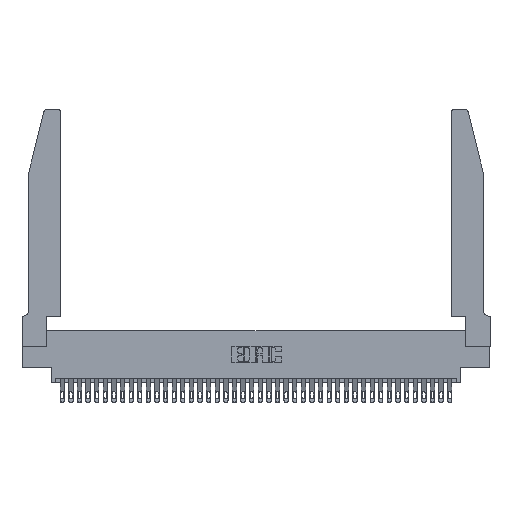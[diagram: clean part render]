
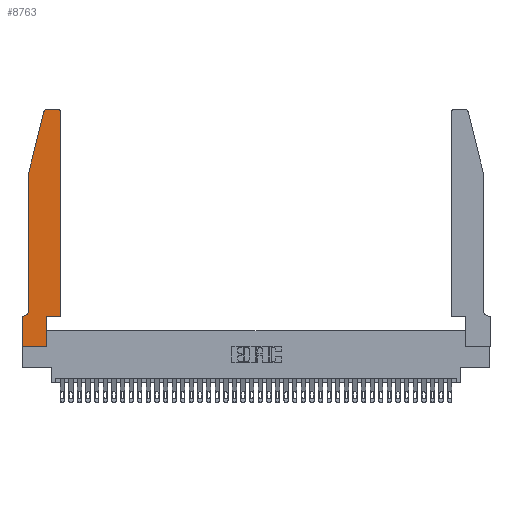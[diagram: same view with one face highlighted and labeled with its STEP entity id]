
A CAD part, top view. The second image highlights one B-rep face of the part: STEP entity #8763.
In plain terms, the highlighted planar face has unit normal (0, 0, 1).
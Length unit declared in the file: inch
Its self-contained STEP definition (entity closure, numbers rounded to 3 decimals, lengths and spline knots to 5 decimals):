
#928 = CARTESIAN_POINT ( 'NONE',  ( 0., 0., 0.37 ) ) ;
#1356 = DIRECTION ( 'NONE',  ( 0., 0., -1. ) ) ;
#1429 = CARTESIAN_POINT ( 'NONE',  ( 0.4505, 0.35, 0.37 ) ) ;
#1814 = EDGE_CURVE ( 'NONE', #34689, #28188, #25560, .T. ) ;
#1971 = AXIS2_PLACEMENT_3D ( 'NONE', #34508, #29140, #38449 ) ;
#2319 = CARTESIAN_POINT ( 'NONE',  ( 0.0755, 0.42, 0.37 ) ) ;
#2362 = VERTEX_POINT ( 'NONE', #7600 ) ;
#2422 = VECTOR ( 'NONE', #18230, 39.37008 ) ;
#2549 = DIRECTION ( 'NONE',  ( 1., 0., 0. ) ) ;
#3381 = ORIENTED_EDGE ( 'NONE', *, *, #33656, .T. ) ;
#3677 = CARTESIAN_POINT ( 'NONE',  ( 0.0755, 2., 0.37 ) ) ;
#3702 = LINE ( 'NONE', #26483, #21016 ) ;
#3932 = VERTEX_POINT ( 'NONE', #34765 ) ;
#4881 = DIRECTION ( 'NONE',  ( 0., -1., 0. ) ) ;
#5626 = LINE ( 'NONE', #1429, #12023 ) ;
#5709 = CARTESIAN_POINT ( 'NONE',  ( 0.4505, 0.35, 0.37 ) ) ;
#5847 = LINE ( 'NONE', #13348, #21200 ) ;
#5885 = CARTESIAN_POINT ( 'NONE',  ( 0., 0., 0.37 ) ) ;
#6052 = CARTESIAN_POINT ( 'NONE',  ( 0.4505, 2.72, 0.37 ) ) ;
#7284 = LINE ( 'NONE', #30276, #17202 ) ;
#7340 = ORIENTED_EDGE ( 'NONE', *, *, #1814, .T. ) ;
#7600 = CARTESIAN_POINT ( 'NONE',  ( 0.2865, 0.35, 0.37 ) ) ;
#8123 = VERTEX_POINT ( 'NONE', #32696 ) ;
#8763 = ADVANCED_FACE ( 'NONE', ( #14436 ), #27932, .T. ) ;
#9829 = AXIS2_PLACEMENT_3D ( 'NONE', #21479, #21331, #2549 ) ;
#9899 = VERTEX_POINT ( 'NONE', #20665 ) ;
#9906 = CIRCLE ( 'NONE', #1971, 0.03 ) ;
#10089 = DIRECTION ( 'NONE',  ( -1., 0., 0. ) ) ;
#10095 = EDGE_CURVE ( 'NONE', #28188, #8123, #24224, .T. ) ;
#10855 = VERTEX_POINT ( 'NONE', #20521 ) ;
#12023 = VECTOR ( 'NONE', #17586, 39.37008 ) ;
#13348 = CARTESIAN_POINT ( 'NONE',  ( 0.2865, 0.35, 0.37 ) ) ;
#13913 = DIRECTION ( 'NONE',  ( -1., 0., 0. ) ) ;
#14436 = FACE_OUTER_BOUND ( 'NONE', #33618, .T. ) ;
#14714 = AXIS2_PLACEMENT_3D ( 'NONE', #16845, #1356, #13913 ) ;
#14833 = AXIS2_PLACEMENT_3D ( 'NONE', #21445, #30648, #21156 ) ;
#15311 = LINE ( 'NONE', #30429, #16774 ) ;
#16774 = VECTOR ( 'NONE', #39851, 39.37008 ) ;
#16806 = ORIENTED_EDGE ( 'NONE', *, *, #36783, .T. ) ;
#16845 = CARTESIAN_POINT ( 'NONE',  ( 0.0055, 0.42, 0.37 ) ) ;
#17202 = VECTOR ( 'NONE', #4881, 39.37008 ) ;
#17586 = DIRECTION ( 'NONE',  ( 1., 0., 0. ) ) ;
#17778 = VECTOR ( 'NONE', #37855, 39.37008 ) ;
#18230 = DIRECTION ( 'NONE',  ( 0., -1., 0. ) ) ;
#18361 = ORIENTED_EDGE ( 'NONE', *, *, #36047, .T. ) ;
#19461 = ORIENTED_EDGE ( 'NONE', *, *, #10095, .T. ) ;
#20137 = DIRECTION ( 'NONE',  ( 0., 1., 0. ) ) ;
#20521 = CARTESIAN_POINT ( 'NONE',  ( 0.0055, 0.35, 0.37 ) ) ;
#20665 = CARTESIAN_POINT ( 'NONE',  ( 0.4205, 2.75, 0.37 ) ) ;
#21016 = VECTOR ( 'NONE', #20137, 39.37008 ) ;
#21137 = CARTESIAN_POINT ( 'NONE',  ( 0.284, 2.75, 0.37 ) ) ;
#21156 = DIRECTION ( 'NONE',  ( 1., 0., 0. ) ) ;
#21200 = VECTOR ( 'NONE', #31905, 39.37008 ) ;
#21331 = DIRECTION ( 'NONE',  ( 0., 0., 1. ) ) ;
#21390 = EDGE_CURVE ( 'NONE', #3932, #38635, #26512, .T. ) ;
#21445 = CARTESIAN_POINT ( 'NONE',  ( 0., 0.35, 0.37 ) ) ;
#21479 = CARTESIAN_POINT ( 'NONE',  ( 0.4205, 2.72, 0.37 ) ) ;
#22908 = EDGE_CURVE ( 'NONE', #29780, #9899, #26357, .T. ) ;
#23590 = ORIENTED_EDGE ( 'NONE', *, *, #24168, .T. ) ;
#24168 = EDGE_CURVE ( 'NONE', #31414, #3932, #9906, .T. ) ;
#24224 = LINE ( 'NONE', #5885, #17778 ) ;
#24580 = VECTOR ( 'NONE', #26044, 39.37008 ) ;
#25560 = LINE ( 'NONE', #37083, #2422 ) ;
#26044 = DIRECTION ( 'NONE',  ( -0.239, -0.971, 0. ) ) ;
#26164 = CIRCLE ( 'NONE', #14714, 0.07 ) ;
#26357 = CIRCLE ( 'NONE', #9829, 0.03 ) ;
#26483 = CARTESIAN_POINT ( 'NONE',  ( 0.4505, 0.35, 0.37 ) ) ;
#26512 = LINE ( 'NONE', #32524, #24580 ) ;
#26565 = EDGE_CURVE ( 'NONE', #10855, #34689, #15311, .T. ) ;
#27119 = EDGE_CURVE ( 'NONE', #38635, #28354, #7284, .T. ) ;
#27932 = PLANE ( 'NONE',  #14833 ) ;
#28188 = VERTEX_POINT ( 'NONE', #928 ) ;
#28354 = VERTEX_POINT ( 'NONE', #2319 ) ;
#29140 = DIRECTION ( 'NONE',  ( 0., 0., 1. ) ) ;
#29544 = VECTOR ( 'NONE', #10089, 39.37008 ) ;
#29780 = VERTEX_POINT ( 'NONE', #6052 ) ;
#30276 = CARTESIAN_POINT ( 'NONE',  ( 0.0755, 2., 0.37 ) ) ;
#30429 = CARTESIAN_POINT ( 'NONE',  ( 0.0755, 0.35, 0.37 ) ) ;
#30648 = DIRECTION ( 'NONE',  ( 0., 0., 1. ) ) ;
#31414 = VERTEX_POINT ( 'NONE', #21137 ) ;
#31905 = DIRECTION ( 'NONE',  ( 0., 1., 0. ) ) ;
#32524 = CARTESIAN_POINT ( 'NONE',  ( 0.0755, 2., 0.37 ) ) ;
#32612 = EDGE_CURVE ( 'NONE', #28354, #10855, #26164, .T. ) ;
#32696 = CARTESIAN_POINT ( 'NONE',  ( 0.2865, 0., 0.37 ) ) ;
#33618 = EDGE_LOOP ( 'NONE', ( #3381, #23590, #40370, #39587, #40609, #39609, #7340, #19461, #39783, #16806, #18361, #34309 ) ) ;
#33656 = EDGE_CURVE ( 'NONE', #9899, #31414, #33959, .T. ) ;
#33959 = LINE ( 'NONE', #39004, #29544 ) ;
#34309 = ORIENTED_EDGE ( 'NONE', *, *, #22908, .T. ) ;
#34508 = CARTESIAN_POINT ( 'NONE',  ( 0.284, 2.72, 0.37 ) ) ;
#34689 = VERTEX_POINT ( 'NONE', #40341 ) ;
#34765 = CARTESIAN_POINT ( 'NONE',  ( 0.25487, 2.72718, 0.37 ) ) ;
#36047 = EDGE_CURVE ( 'NONE', #39090, #29780, #3702, .T. ) ;
#36783 = EDGE_CURVE ( 'NONE', #2362, #39090, #5626, .T. ) ;
#37083 = CARTESIAN_POINT ( 'NONE',  ( 0., 0., 0.37 ) ) ;
#37855 = DIRECTION ( 'NONE',  ( 1., 0., 0. ) ) ;
#38449 = DIRECTION ( 'NONE',  ( 1., 0., 0. ) ) ;
#38635 = VERTEX_POINT ( 'NONE', #3677 ) ;
#39004 = CARTESIAN_POINT ( 'NONE',  ( 0.2605, 2.75, 0.37 ) ) ;
#39090 = VERTEX_POINT ( 'NONE', #5709 ) ;
#39587 = ORIENTED_EDGE ( 'NONE', *, *, #27119, .T. ) ;
#39609 = ORIENTED_EDGE ( 'NONE', *, *, #26565, .T. ) ;
#39783 = ORIENTED_EDGE ( 'NONE', *, *, #39873, .T. ) ;
#39851 = DIRECTION ( 'NONE',  ( -1., 0., 0. ) ) ;
#39873 = EDGE_CURVE ( 'NONE', #8123, #2362, #5847, .T. ) ;
#40341 = CARTESIAN_POINT ( 'NONE',  ( 0., 0.35, 0.37 ) ) ;
#40370 = ORIENTED_EDGE ( 'NONE', *, *, #21390, .T. ) ;
#40609 = ORIENTED_EDGE ( 'NONE', *, *, #32612, .T. ) ;
